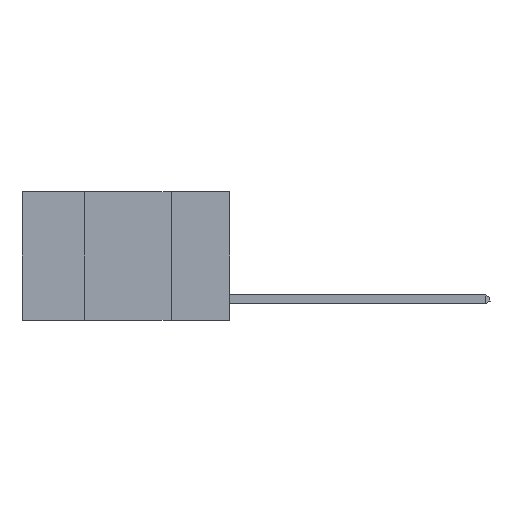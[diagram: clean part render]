
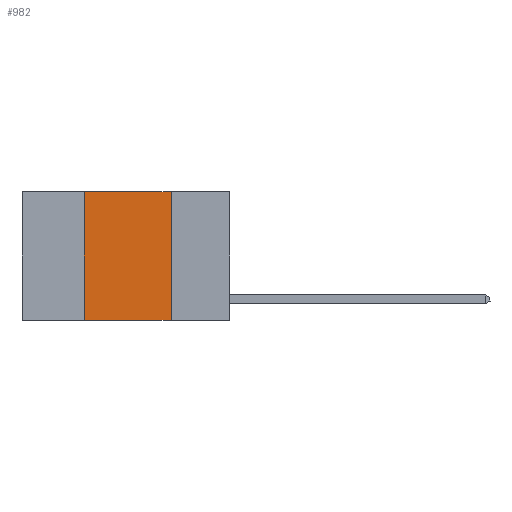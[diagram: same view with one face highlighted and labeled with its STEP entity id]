
A CAD part, left-side view. The second image highlights one B-rep face of the part: STEP entity #982.
In plain terms, the highlighted planar face has unit normal (-1, 0, 0).
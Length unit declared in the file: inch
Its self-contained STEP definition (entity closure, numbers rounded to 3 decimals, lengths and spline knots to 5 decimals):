
#631 = CARTESIAN_POINT ( 'NONE',  ( 0., 0.6, 0. ) ) ;
#707 = LINE ( 'NONE', #4431, #5659 ) ;
#979 = VERTEX_POINT ( 'NONE', #7703 ) ;
#982 = ADVANCED_FACE ( 'NONE', ( #11400 ), #3433, .F. ) ;
#1123 = CARTESIAN_POINT ( 'NONE',  ( 0., 0.6, 0. ) ) ;
#1325 = CARTESIAN_POINT ( 'NONE',  ( 0., 0.6, -0.37 ) ) ;
#2134 = AXIS2_PLACEMENT_3D ( 'NONE', #631, #3376, #10800 ) ;
#3147 = CARTESIAN_POINT ( 'NONE',  ( 0., 0.42, 0. ) ) ;
#3268 = CARTESIAN_POINT ( 'NONE',  ( 0., 0.17, -0.37 ) ) ;
#3376 = DIRECTION ( 'NONE',  ( 1., 0., 0. ) ) ;
#3389 = LINE ( 'NONE', #1325, #11317 ) ;
#3433 = PLANE ( 'NONE',  #2134 ) ;
#4431 = CARTESIAN_POINT ( 'NONE',  ( 0., 0.42, 0. ) ) ;
#5095 = DIRECTION ( 'NONE',  ( 0., -1., 0. ) ) ;
#5337 = DIRECTION ( 'NONE',  ( 0., 0., -1. ) ) ;
#5587 = EDGE_CURVE ( 'NONE', #8437, #6687, #3389, .T. ) ;
#5659 = VECTOR ( 'NONE', #11487, 39.37008 ) ;
#6227 = VECTOR ( 'NONE', #5337, 39.37008 ) ;
#6517 = CARTESIAN_POINT ( 'NONE',  ( 0., 0.42, -0.37 ) ) ;
#6687 = VERTEX_POINT ( 'NONE', #3268 ) ;
#7022 = VECTOR ( 'NONE', #8327, 39.37008 ) ;
#7541 = ORIENTED_EDGE ( 'NONE', *, *, #10137, .F. ) ;
#7703 = CARTESIAN_POINT ( 'NONE',  ( 0., 0.17, 0. ) ) ;
#8327 = DIRECTION ( 'NONE',  ( 0., -1., 0. ) ) ;
#8335 = EDGE_LOOP ( 'NONE', ( #10490, #8747, #7541, #11079 ) ) ;
#8437 = VERTEX_POINT ( 'NONE', #6517 ) ;
#8747 = ORIENTED_EDGE ( 'NONE', *, *, #10211, .F. ) ;
#9385 = VERTEX_POINT ( 'NONE', #3147 ) ;
#9411 = LINE ( 'NONE', #1123, #7022 ) ;
#10066 = EDGE_CURVE ( 'NONE', #979, #6687, #10926, .T. ) ;
#10077 = CARTESIAN_POINT ( 'NONE',  ( 0., 0.17, 0. ) ) ;
#10137 = EDGE_CURVE ( 'NONE', #8437, #9385, #707, .T. ) ;
#10211 = EDGE_CURVE ( 'NONE', #9385, #979, #9411, .T. ) ;
#10490 = ORIENTED_EDGE ( 'NONE', *, *, #10066, .F. ) ;
#10800 = DIRECTION ( 'NONE',  ( 0., 0., -1. ) ) ;
#10926 = LINE ( 'NONE', #10077, #6227 ) ;
#11079 = ORIENTED_EDGE ( 'NONE', *, *, #5587, .T. ) ;
#11317 = VECTOR ( 'NONE', #5095, 39.37008 ) ;
#11400 = FACE_OUTER_BOUND ( 'NONE', #8335, .T. ) ;
#11487 = DIRECTION ( 'NONE',  ( 0., 0., 1. ) ) ;
